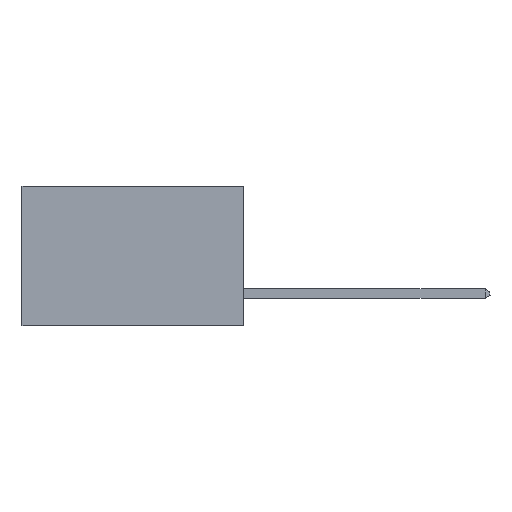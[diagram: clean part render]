
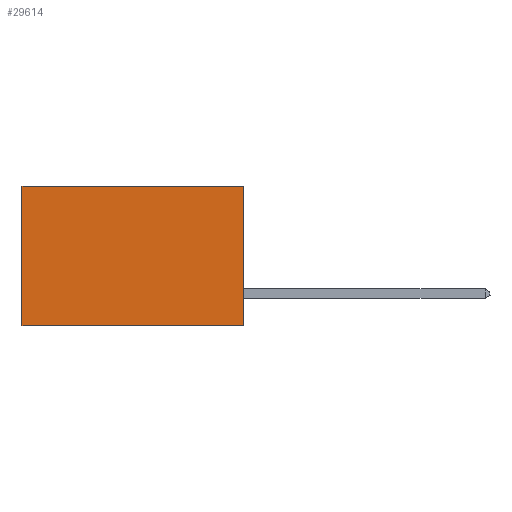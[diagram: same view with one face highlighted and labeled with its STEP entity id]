
A CAD part, left-side view. The second image highlights one B-rep face of the part: STEP entity #29614.
In plain terms, the highlighted planar face has unit normal (-1, 0, 0).
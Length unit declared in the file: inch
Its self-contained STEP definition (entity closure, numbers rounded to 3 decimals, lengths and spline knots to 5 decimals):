
#1130 = ORIENTED_EDGE ( 'NONE', *, *, #8825, .F. ) ;
#2341 = ORIENTED_EDGE ( 'NONE', *, *, #5196, .T. ) ;
#2981 = EDGE_CURVE ( 'NONE', #21497, #11302, #31390, .T. ) ;
#3633 = CARTESIAN_POINT ( 'NONE',  ( 0.277, 0.59, 0. ) ) ;
#3822 = FACE_OUTER_BOUND ( 'NONE', #4756, .T. ) ;
#3963 = DIRECTION ( 'NONE',  ( 0., 0., -1. ) ) ;
#4756 = EDGE_LOOP ( 'NONE', ( #20620, #22127, #1130, #2341 ) ) ;
#5196 = EDGE_CURVE ( 'NONE', #9082, #21497, #21390, .T. ) ;
#6102 = CARTESIAN_POINT ( 'NONE',  ( 0.277, 0., -0.37 ) ) ;
#6343 = CARTESIAN_POINT ( 'NONE',  ( 0.277, 0., -0.37 ) ) ;
#8644 = DIRECTION ( 'NONE',  ( 0., 0., -1. ) ) ;
#8825 = EDGE_CURVE ( 'NONE', #9082, #13658, #25146, .T. ) ;
#9082 = VERTEX_POINT ( 'NONE', #14216 ) ;
#11302 = VERTEX_POINT ( 'NONE', #20098 ) ;
#13658 = VERTEX_POINT ( 'NONE', #28169 ) ;
#14216 = CARTESIAN_POINT ( 'NONE',  ( 0.277, 0., 0. ) ) ;
#15872 = LINE ( 'NONE', #6343, #28037 ) ;
#18340 = CARTESIAN_POINT ( 'NONE',  ( 0.277, 0., -0.37 ) ) ;
#19677 = DIRECTION ( 'NONE',  ( 0., 0., -1. ) ) ;
#19780 = DIRECTION ( 'NONE',  ( 0., 1., 0. ) ) ;
#20098 = CARTESIAN_POINT ( 'NONE',  ( 0.277, 0.59, -0.37 ) ) ;
#20620 = ORIENTED_EDGE ( 'NONE', *, *, #2981, .T. ) ;
#20857 = PLANE ( 'NONE',  #26785 ) ;
#21390 = LINE ( 'NONE', #25413, #26342 ) ;
#21497 = VERTEX_POINT ( 'NONE', #3633 ) ;
#22127 = ORIENTED_EDGE ( 'NONE', *, *, #22831, .F. ) ;
#22831 = EDGE_CURVE ( 'NONE', #13658, #11302, #15872, .T. ) ;
#23324 = VECTOR ( 'NONE', #19677, 39.37008 ) ;
#23338 = DIRECTION ( 'NONE',  ( 1., 0., 0. ) ) ;
#24364 = VECTOR ( 'NONE', #3963, 39.37008 ) ;
#25146 = LINE ( 'NONE', #18340, #24364 ) ;
#25413 = CARTESIAN_POINT ( 'NONE',  ( 0.277, 0., 0. ) ) ;
#26342 = VECTOR ( 'NONE', #19780, 39.37008 ) ;
#26785 = AXIS2_PLACEMENT_3D ( 'NONE', #6102, #23338, #8644 ) ;
#28037 = VECTOR ( 'NONE', #28527, 39.37008 ) ;
#28169 = CARTESIAN_POINT ( 'NONE',  ( 0.277, 0., -0.37 ) ) ;
#28527 = DIRECTION ( 'NONE',  ( 0., 1., 0. ) ) ;
#29614 = ADVANCED_FACE ( 'NONE', ( #3822 ), #20857, .F. ) ;
#31377 = CARTESIAN_POINT ( 'NONE',  ( 0.277, 0.59, -0.37 ) ) ;
#31390 = LINE ( 'NONE', #31377, #23324 ) ;
